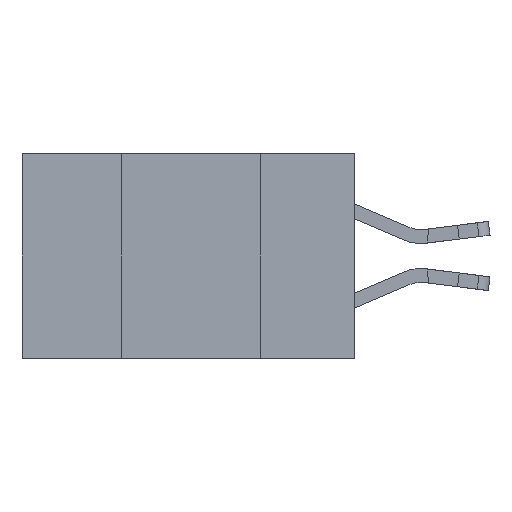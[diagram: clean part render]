
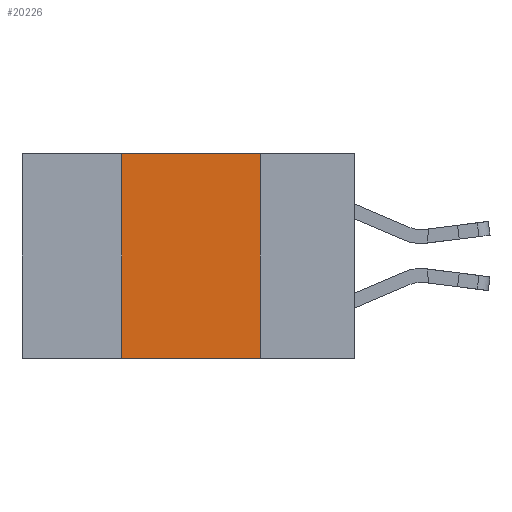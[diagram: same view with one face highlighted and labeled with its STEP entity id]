
A CAD part, left-side view. The second image highlights one B-rep face of the part: STEP entity #20226.
In plain terms, the highlighted planar face has unit normal (-1, 0, 0).
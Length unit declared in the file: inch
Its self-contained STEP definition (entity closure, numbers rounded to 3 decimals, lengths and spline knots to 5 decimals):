
#912 = CARTESIAN_POINT ( 'NONE',  ( 0., 0.17, 0. ) ) ;
#1209 = ORIENTED_EDGE ( 'NONE', *, *, #8178, .F. ) ;
#2057 = CARTESIAN_POINT ( 'NONE',  ( 0., 0.17, 0. ) ) ;
#2476 = CARTESIAN_POINT ( 'NONE',  ( 0., 0.42, 0. ) ) ;
#2631 = ORIENTED_EDGE ( 'NONE', *, *, #10341, .F. ) ;
#3172 = LINE ( 'NONE', #13490, #6501 ) ;
#3667 = LINE ( 'NONE', #2476, #7471 ) ;
#3962 = LINE ( 'NONE', #2057, #11543 ) ;
#3973 = DIRECTION ( 'NONE',  ( 1., 0., 0. ) ) ;
#4828 = AXIS2_PLACEMENT_3D ( 'NONE', #13648, #3973, #15217 ) ;
#5421 = ORIENTED_EDGE ( 'NONE', *, *, #19283, .F. ) ;
#5991 = VERTEX_POINT ( 'NONE', #912 ) ;
#6178 = DIRECTION ( 'NONE',  ( 0., 0., 1. ) ) ;
#6501 = VECTOR ( 'NONE', #13531, 39.37008 ) ;
#7092 = EDGE_CURVE ( 'NONE', #20558, #19089, #3172, .T. ) ;
#7471 = VECTOR ( 'NONE', #6178, 39.37008 ) ;
#8178 = EDGE_CURVE ( 'NONE', #20558, #13837, #3667, .T. ) ;
#9801 = FACE_OUTER_BOUND ( 'NONE', #14403, .T. ) ;
#9827 = DIRECTION ( 'NONE',  ( 0., -1., 0. ) ) ;
#10339 = PLANE ( 'NONE',  #4828 ) ;
#10341 = EDGE_CURVE ( 'NONE', #5991, #19089, #3962, .T. ) ;
#10459 = CARTESIAN_POINT ( 'NONE',  ( 0., 0.42, 0. ) ) ;
#10850 = VECTOR ( 'NONE', #9827, 39.37008 ) ;
#11351 = LINE ( 'NONE', #17751, #10850 ) ;
#11543 = VECTOR ( 'NONE', #16530, 39.37008 ) ;
#13490 = CARTESIAN_POINT ( 'NONE',  ( 0., 0.6, -0.37 ) ) ;
#13531 = DIRECTION ( 'NONE',  ( 0., -1., 0. ) ) ;
#13648 = CARTESIAN_POINT ( 'NONE',  ( 0., 0.6, 0. ) ) ;
#13837 = VERTEX_POINT ( 'NONE', #10459 ) ;
#14403 = EDGE_LOOP ( 'NONE', ( #2631, #5421, #1209, #17622 ) ) ;
#15217 = DIRECTION ( 'NONE',  ( 0., 0., -1. ) ) ;
#15752 = CARTESIAN_POINT ( 'NONE',  ( 0., 0.17, -0.37 ) ) ;
#16530 = DIRECTION ( 'NONE',  ( 0., 0., -1. ) ) ;
#17622 = ORIENTED_EDGE ( 'NONE', *, *, #7092, .T. ) ;
#17751 = CARTESIAN_POINT ( 'NONE',  ( 0., 0.6, 0. ) ) ;
#19089 = VERTEX_POINT ( 'NONE', #15752 ) ;
#19254 = CARTESIAN_POINT ( 'NONE',  ( 0., 0.42, -0.37 ) ) ;
#19283 = EDGE_CURVE ( 'NONE', #13837, #5991, #11351, .T. ) ;
#20226 = ADVANCED_FACE ( 'NONE', ( #9801 ), #10339, .F. ) ;
#20558 = VERTEX_POINT ( 'NONE', #19254 ) ;
